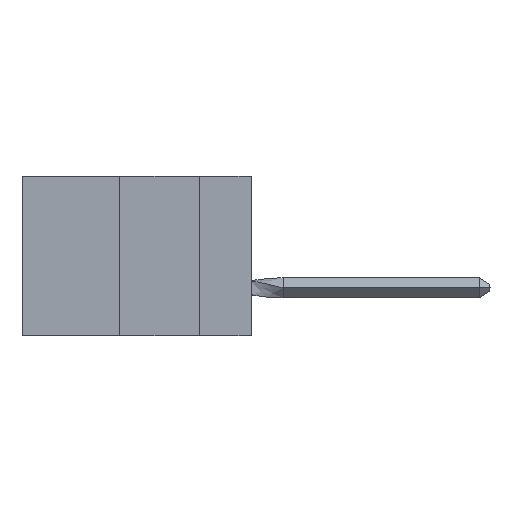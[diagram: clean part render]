
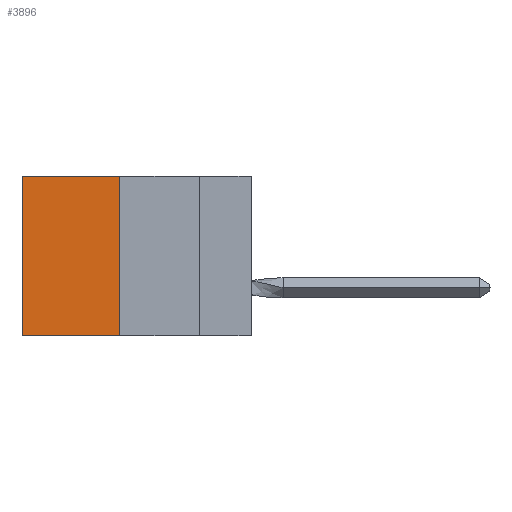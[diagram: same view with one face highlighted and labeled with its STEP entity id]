
A CAD part, left-side view. The second image highlights one B-rep face of the part: STEP entity #3896.
In plain terms, the highlighted planar face has unit normal (-1, 0, 0).
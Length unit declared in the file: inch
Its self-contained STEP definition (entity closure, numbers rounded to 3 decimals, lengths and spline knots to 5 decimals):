
#175 = CARTESIAN_POINT ( 'NONE',  ( 0.305, 0.72, -0.5 ) ) ;
#255 = VECTOR ( 'NONE', #6805, 39.37008 ) ;
#637 = VERTEX_POINT ( 'NONE', #175 ) ;
#1368 = EDGE_CURVE ( 'NONE', #9285, #11044, #7707, .T. ) ;
#1469 = DIRECTION ( 'NONE',  ( 0., 0., -1. ) ) ;
#1745 = CARTESIAN_POINT ( 'NONE',  ( 0.305, 0.413, -0.5 ) ) ;
#2135 = LINE ( 'NONE', #6742, #3782 ) ;
#2598 = CARTESIAN_POINT ( 'NONE',  ( 0.305, 0.413, -0.5 ) ) ;
#3677 = DIRECTION ( 'NONE',  ( 0., 0., -1. ) ) ;
#3730 = EDGE_CURVE ( 'NONE', #11044, #637, #11696, .T. ) ;
#3782 = VECTOR ( 'NONE', #1469, 39.37008 ) ;
#3896 = ADVANCED_FACE ( 'NONE', ( #11038 ), #10795, .F. ) ;
#4285 = CARTESIAN_POINT ( 'NONE',  ( 0.305, 0.72, 0. ) ) ;
#6702 = CARTESIAN_POINT ( 'NONE',  ( 0.305, 0.413, 0. ) ) ;
#6742 = CARTESIAN_POINT ( 'NONE',  ( 0.305, 0.413, -0.5 ) ) ;
#6805 = DIRECTION ( 'NONE',  ( 0., 1., 0. ) ) ;
#7173 = ORIENTED_EDGE ( 'NONE', *, *, #10651, .F. ) ;
#7707 = LINE ( 'NONE', #11839, #13500 ) ;
#9285 = VERTEX_POINT ( 'NONE', #6702 ) ;
#9370 = LINE ( 'NONE', #2598, #255 ) ;
#9427 = VERTEX_POINT ( 'NONE', #1745 ) ;
#9632 = DIRECTION ( 'NONE',  ( 0., 0., -1. ) ) ;
#9718 = CARTESIAN_POINT ( 'NONE',  ( 0.305, 0.413, -0.5 ) ) ;
#9756 = AXIS2_PLACEMENT_3D ( 'NONE', #9718, #9815, #9632 ) ;
#9815 = DIRECTION ( 'NONE',  ( 1., 0., 0. ) ) ;
#10255 = ORIENTED_EDGE ( 'NONE', *, *, #3730, .T. ) ;
#10599 = ORIENTED_EDGE ( 'NONE', *, *, #11975, .F. ) ;
#10651 = EDGE_CURVE ( 'NONE', #9285, #9427, #2135, .T. ) ;
#10795 = PLANE ( 'NONE',  #9756 ) ;
#11038 = FACE_OUTER_BOUND ( 'NONE', #12246, .T. ) ;
#11044 = VERTEX_POINT ( 'NONE', #4285 ) ;
#11582 = ORIENTED_EDGE ( 'NONE', *, *, #1368, .T. ) ;
#11696 = LINE ( 'NONE', #12049, #12334 ) ;
#11839 = CARTESIAN_POINT ( 'NONE',  ( 0.305, 0.413, 0. ) ) ;
#11964 = DIRECTION ( 'NONE',  ( 0., 1., 0. ) ) ;
#11975 = EDGE_CURVE ( 'NONE', #9427, #637, #9370, .T. ) ;
#12049 = CARTESIAN_POINT ( 'NONE',  ( 0.305, 0.72, -0.5 ) ) ;
#12246 = EDGE_LOOP ( 'NONE', ( #10255, #10599, #7173, #11582 ) ) ;
#12334 = VECTOR ( 'NONE', #3677, 39.37008 ) ;
#13500 = VECTOR ( 'NONE', #11964, 39.37008 ) ;
